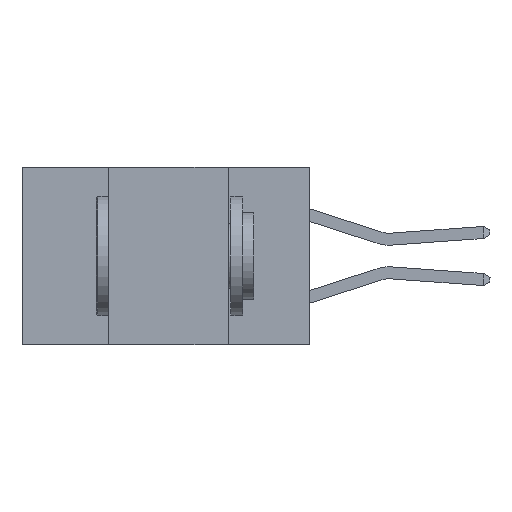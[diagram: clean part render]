
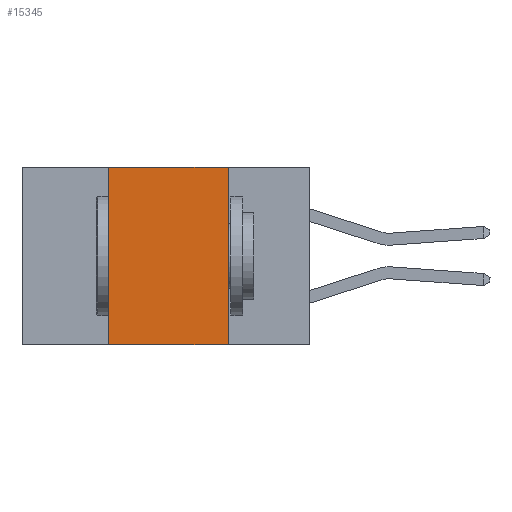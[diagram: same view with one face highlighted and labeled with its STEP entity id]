
A CAD part, left-side view. The second image highlights one B-rep face of the part: STEP entity #15345.
In plain terms, the highlighted planar face has unit normal (-1, 0, 0).
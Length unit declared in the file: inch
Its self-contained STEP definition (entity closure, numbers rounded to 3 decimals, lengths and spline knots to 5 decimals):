
#1780 = AXIS2_PLACEMENT_3D ( 'NONE', #18668, #20716, #8603 ) ;
#1980 = ORIENTED_EDGE ( 'NONE', *, *, #9485, .F. ) ;
#2165 = ORIENTED_EDGE ( 'NONE', *, *, #4995, .F. ) ;
#2477 = ORIENTED_EDGE ( 'NONE', *, *, #13696, .F. ) ;
#2925 = DIRECTION ( 'NONE',  ( 0., 0., -1. ) ) ;
#2939 = ORIENTED_EDGE ( 'NONE', *, *, #14872, .T. ) ;
#3417 = DIRECTION ( 'NONE',  ( 0., -1., 0. ) ) ;
#4440 = PLANE ( 'NONE',  #1780 ) ;
#4699 = VECTOR ( 'NONE', #3417, 39.37008 ) ;
#4995 = EDGE_CURVE ( 'NONE', #26206, #19353, #20916, .T. ) ;
#5211 = CARTESIAN_POINT ( 'NONE',  ( 0., 0.17, -0.37 ) ) ;
#6962 = LINE ( 'NONE', #12565, #17075 ) ;
#7500 = EDGE_LOOP ( 'NONE', ( #1980, #2165, #2477, #2939 ) ) ;
#8173 = VERTEX_POINT ( 'NONE', #5211 ) ;
#8603 = DIRECTION ( 'NONE',  ( 0., 0., -1. ) ) ;
#9485 = EDGE_CURVE ( 'NONE', #19353, #8173, #22221, .T. ) ;
#9776 = FACE_OUTER_BOUND ( 'NONE', #7500, .T. ) ;
#9805 = VECTOR ( 'NONE', #20130, 39.37008 ) ;
#11035 = CARTESIAN_POINT ( 'NONE',  ( 0., 0.17, 0. ) ) ;
#11702 = CARTESIAN_POINT ( 'NONE',  ( 0., 0.42, 0. ) ) ;
#12565 = CARTESIAN_POINT ( 'NONE',  ( 0., 0.42, -0.37 ) ) ;
#13696 = EDGE_CURVE ( 'NONE', #24180, #26206, #6962, .T. ) ;
#14872 = EDGE_CURVE ( 'NONE', #24180, #8173, #15150, .T. ) ;
#15150 = LINE ( 'NONE', #16039, #9805 ) ;
#15345 = ADVANCED_FACE ( 'NONE', ( #9776 ), #4440, .F. ) ;
#16039 = CARTESIAN_POINT ( 'NONE',  ( 0., 0.6, -0.37 ) ) ;
#16830 = VECTOR ( 'NONE', #2925, 39.37008 ) ;
#17075 = VECTOR ( 'NONE', #22723, 39.37008 ) ;
#17104 = CARTESIAN_POINT ( 'NONE',  ( 0., 0.17, -0.37 ) ) ;
#17674 = CARTESIAN_POINT ( 'NONE',  ( 0., 0.6, 0. ) ) ;
#18668 = CARTESIAN_POINT ( 'NONE',  ( 0., 0.6, 0. ) ) ;
#18991 = CARTESIAN_POINT ( 'NONE',  ( 0., 0.42, -0.37 ) ) ;
#19353 = VERTEX_POINT ( 'NONE', #11035 ) ;
#20130 = DIRECTION ( 'NONE',  ( 0., -1., 0. ) ) ;
#20716 = DIRECTION ( 'NONE',  ( 1., 0., 0. ) ) ;
#20916 = LINE ( 'NONE', #17674, #4699 ) ;
#22221 = LINE ( 'NONE', #17104, #16830 ) ;
#22723 = DIRECTION ( 'NONE',  ( 0., 0., 1. ) ) ;
#24180 = VERTEX_POINT ( 'NONE', #18991 ) ;
#26206 = VERTEX_POINT ( 'NONE', #11702 ) ;
